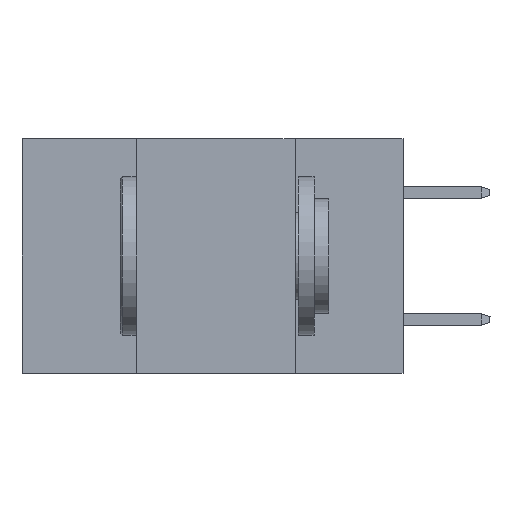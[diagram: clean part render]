
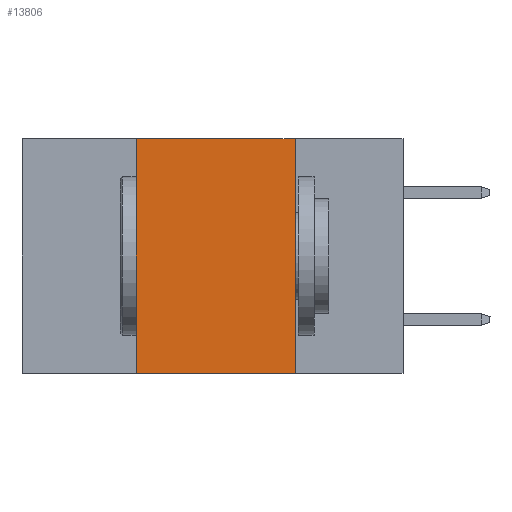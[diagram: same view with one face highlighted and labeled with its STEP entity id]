
A CAD part, left-side view. The second image highlights one B-rep face of the part: STEP entity #13806.
In plain terms, the highlighted planar face has unit normal (-1, 0, 0).
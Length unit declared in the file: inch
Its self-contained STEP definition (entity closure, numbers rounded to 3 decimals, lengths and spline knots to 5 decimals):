
#704 = LINE ( 'NONE', #3637, #13086 ) ;
#765 = VERTEX_POINT ( 'NONE', #2258 ) ;
#1006 = ORIENTED_EDGE ( 'NONE', *, *, #14987, .F. ) ;
#1335 = FACE_OUTER_BOUND ( 'NONE', #8343, .T. ) ;
#1451 = AXIS2_PLACEMENT_3D ( 'NONE', #18708, #2466, #6942 ) ;
#2258 = CARTESIAN_POINT ( 'NONE',  ( 0., 0.17, 0. ) ) ;
#2466 = DIRECTION ( 'NONE',  ( 1., 0., 0. ) ) ;
#2824 = VERTEX_POINT ( 'NONE', #10940 ) ;
#3637 = CARTESIAN_POINT ( 'NONE',  ( 0., 0.17, 0. ) ) ;
#3651 = EDGE_CURVE ( 'NONE', #10649, #2824, #7070, .T. ) ;
#3973 = PLANE ( 'NONE',  #1451 ) ;
#3986 = CARTESIAN_POINT ( 'NONE',  ( 0., 0.42, 0. ) ) ;
#4291 = VERTEX_POINT ( 'NONE', #12562 ) ;
#5388 = VECTOR ( 'NONE', #11798, 39.37008 ) ;
#5621 = DIRECTION ( 'NONE',  ( 0., -1., 0. ) ) ;
#5727 = VECTOR ( 'NONE', #6857, 39.37008 ) ;
#5803 = ORIENTED_EDGE ( 'NONE', *, *, #17049, .F. ) ;
#5944 = LINE ( 'NONE', #9109, #5388 ) ;
#6857 = DIRECTION ( 'NONE',  ( 0., 0., 1. ) ) ;
#6942 = DIRECTION ( 'NONE',  ( 0., 0., -1. ) ) ;
#7070 = LINE ( 'NONE', #12929, #14085 ) ;
#8343 = EDGE_LOOP ( 'NONE', ( #1006, #13495, #5803, #10642 ) ) ;
#9109 = CARTESIAN_POINT ( 'NONE',  ( 0., 0.6, 0. ) ) ;
#10642 = ORIENTED_EDGE ( 'NONE', *, *, #3651, .T. ) ;
#10649 = VERTEX_POINT ( 'NONE', #14572 ) ;
#10940 = CARTESIAN_POINT ( 'NONE',  ( 0., 0.17, -0.37 ) ) ;
#11798 = DIRECTION ( 'NONE',  ( 0., -1., 0. ) ) ;
#12353 = DIRECTION ( 'NONE',  ( 0., 0., -1. ) ) ;
#12562 = CARTESIAN_POINT ( 'NONE',  ( 0., 0.42, 0. ) ) ;
#12929 = CARTESIAN_POINT ( 'NONE',  ( 0., 0.6, -0.37 ) ) ;
#13086 = VECTOR ( 'NONE', #12353, 39.37008 ) ;
#13495 = ORIENTED_EDGE ( 'NONE', *, *, #16231, .F. ) ;
#13806 = ADVANCED_FACE ( 'NONE', ( #1335 ), #3973, .F. ) ;
#14085 = VECTOR ( 'NONE', #5621, 39.37008 ) ;
#14572 = CARTESIAN_POINT ( 'NONE',  ( 0., 0.42, -0.37 ) ) ;
#14987 = EDGE_CURVE ( 'NONE', #765, #2824, #704, .T. ) ;
#16231 = EDGE_CURVE ( 'NONE', #4291, #765, #5944, .T. ) ;
#17049 = EDGE_CURVE ( 'NONE', #10649, #4291, #17109, .T. ) ;
#17109 = LINE ( 'NONE', #3986, #5727 ) ;
#18708 = CARTESIAN_POINT ( 'NONE',  ( 0., 0.6, 0. ) ) ;
